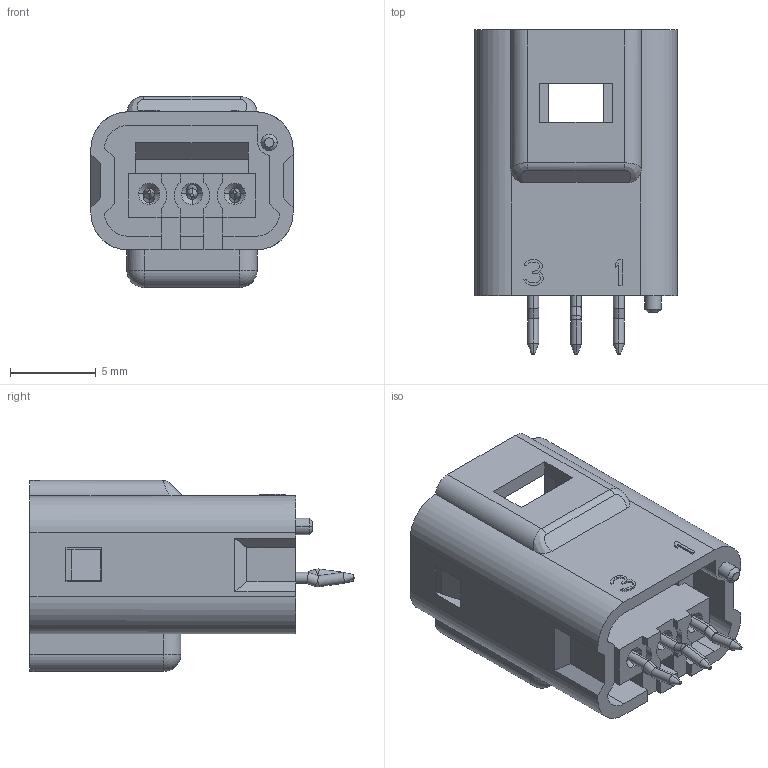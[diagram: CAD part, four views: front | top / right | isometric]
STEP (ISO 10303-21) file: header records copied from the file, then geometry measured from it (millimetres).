
FILE_DESCRIPTION (( 'STEP AP203' ), '1' );
FILE_NAME ('560-003-420-501.STEP', '2020-07-24T16:52:33', ( '' ), ( '' ), 'SwSTEP 2.0', 'SolidWorks 2020', '' );
FILE_SCHEMA (( 'CONFIG_CONTROL_DESIGN' ));
Length unit declared in the file: millimetre
Products named in the file (8): CONTACT_PCB-HEADER-2; FACIAL_SEAL; CONTACT_PCB-HEADER; HOUSING-3POS_PCB-HEADER_ORANGE; 560-003-420-501; CONTACT_PCB-HEADER-1; INTERNAL-WIRE-SEAL-3POS
Assembly tree (7 placements, depth 3):
  560-003-420-501
    560-003-420-501
      HOUSING-3POS_PCB-HEADER_ORANGE
      CONTACT_PCB-HEADER
      CONTACT_PCB-HEADER-1
      CONTACT_PCB-HEADER-2
      INTERNAL-WIRE-SEAL-3POS
      FACIAL_SEAL
Bounding box: 11.8 x 18.9 x 11.15 mm (x, y, z)
Volume: 754.2 mm3; surface area: 2157.4 mm2
Topology: 6 solids, 6 shells, 663 faces, 1680 edges, 1045 vertices
Faces by surface type: plane 398, cylinder 157, cone 54, torus 44, bspline 8, sphere 2
Entity records: 21149 total; most frequent: CARTESIAN_POINT 4288, ORIENTED_EDGE 3356, DIRECTION 3315, EDGE_CURVE 1678, VECTOR 1163, LINE 1163, AXIS2_PLACEMENT_3D 1076, VERTEX_POINT 1045
